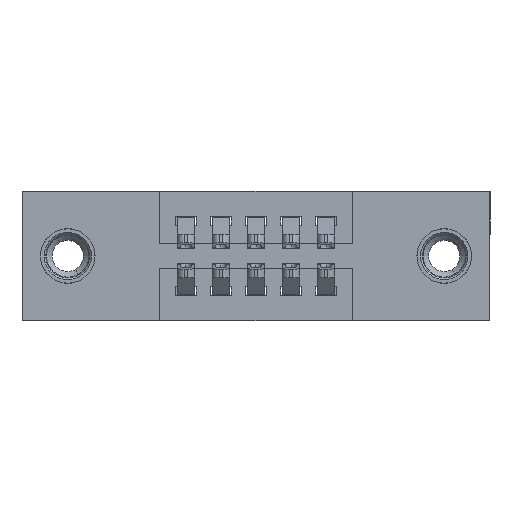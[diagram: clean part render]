
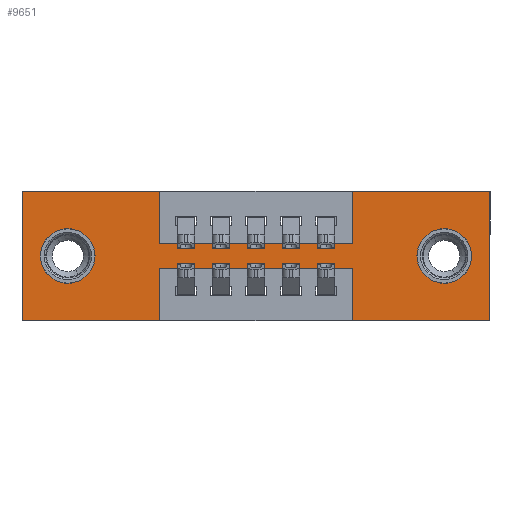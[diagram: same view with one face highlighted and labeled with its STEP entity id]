
A CAD part, front view. The second image highlights one B-rep face of the part: STEP entity #9651.
In plain terms, the highlighted planar face has unit normal (0, -1, 0).
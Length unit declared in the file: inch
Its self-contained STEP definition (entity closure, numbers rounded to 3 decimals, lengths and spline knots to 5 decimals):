
#229 = EDGE_LOOP ( 'NONE', ( #11366, #8792 ) ) ;
#254 = VERTEX_POINT ( 'NONE', #991 ) ;
#632 = FACE_OUTER_BOUND ( 'NONE', #6488, .T. ) ;
#671 = VECTOR ( 'NONE', #4247, 39.37008 ) ;
#933 = DIRECTION ( 'NONE',  ( -1., 0., 0. ) ) ;
#991 = CARTESIAN_POINT ( 'NONE',  ( 0.13, 0., -0.107 ) ) ;
#1004 = CARTESIAN_POINT ( 'NONE',  ( 0.3925, 0., -0.15 ) ) ;
#1120 = DIRECTION ( 'NONE',  ( 0., 1., 0. ) ) ;
#1125 = EDGE_CURVE ( 'NONE', #12646, #8550, #12252, .T. ) ;
#1458 = VERTEX_POINT ( 'NONE', #2628 ) ;
#1534 = ORIENTED_EDGE ( 'NONE', *, *, #6074, .F. ) ;
#1976 = VECTOR ( 'NONE', #12030, 39.37008 ) ;
#2078 = CARTESIAN_POINT ( 'NONE',  ( 0.13, 0., -0.185 ) ) ;
#2145 = LINE ( 'NONE', #2815, #13195 ) ;
#2158 = CARTESIAN_POINT ( 'NONE',  ( 0., 0., -0.37 ) ) ;
#2210 = PLANE ( 'NONE',  #7024 ) ;
#2267 = CARTESIAN_POINT ( 'NONE',  ( 0.9425, 0., -0.37 ) ) ;
#2303 = CARTESIAN_POINT ( 'NONE',  ( 1.205, 0., -0.185 ) ) ;
#2344 = ORIENTED_EDGE ( 'NONE', *, *, #8159, .F. ) ;
#2494 = VERTEX_POINT ( 'NONE', #3335 ) ;
#2552 = CARTESIAN_POINT ( 'NONE',  ( 0.13, 0., -0.185 ) ) ;
#2619 = CARTESIAN_POINT ( 'NONE',  ( 0.9425, 0., -0.37 ) ) ;
#2628 = CARTESIAN_POINT ( 'NONE',  ( 0.9425, 0., 0. ) ) ;
#2689 = CARTESIAN_POINT ( 'NONE',  ( 0., 0., -0.37 ) ) ;
#2693 = VECTOR ( 'NONE', #6007, 39.37008 ) ;
#2753 = ORIENTED_EDGE ( 'NONE', *, *, #3993, .F. ) ;
#2815 = CARTESIAN_POINT ( 'NONE',  ( 0.9425, 0., 0. ) ) ;
#2883 = CARTESIAN_POINT ( 'NONE',  ( 1.335, 0., -0.37 ) ) ;
#2893 = CARTESIAN_POINT ( 'NONE',  ( 0.13, 0., -0.263 ) ) ;
#2977 = VERTEX_POINT ( 'NONE', #6370 ) ;
#3029 = LINE ( 'NONE', #7100, #2693 ) ;
#3079 = VERTEX_POINT ( 'NONE', #12874 ) ;
#3143 = DIRECTION ( 'NONE',  ( 0., 0., 1. ) ) ;
#3152 = CARTESIAN_POINT ( 'NONE',  ( 0., 0., 0. ) ) ;
#3208 = CARTESIAN_POINT ( 'NONE',  ( 0.3925, 0., 0. ) ) ;
#3283 = LINE ( 'NONE', #7606, #5540 ) ;
#3298 = LINE ( 'NONE', #7542, #11921 ) ;
#3320 = DIRECTION ( 'NONE',  ( 0., 0., -1. ) ) ;
#3335 = CARTESIAN_POINT ( 'NONE',  ( 0.9425, 0., -0.22 ) ) ;
#3363 = DIRECTION ( 'NONE',  ( 0., 0., -1. ) ) ;
#3390 = VECTOR ( 'NONE', #10208, 39.37008 ) ;
#3630 = DIRECTION ( 'NONE',  ( 0., 0., 1. ) ) ;
#3690 = VERTEX_POINT ( 'NONE', #5334 ) ;
#3976 = VECTOR ( 'NONE', #13408, 39.37008 ) ;
#3981 = ORIENTED_EDGE ( 'NONE', *, *, #12559, .F. ) ;
#3993 = EDGE_CURVE ( 'NONE', #10356, #2977, #3029, .T. ) ;
#4084 = VERTEX_POINT ( 'NONE', #2883 ) ;
#4247 = DIRECTION ( 'NONE',  ( 0., 0., 1. ) ) ;
#4345 = VECTOR ( 'NONE', #7446, 39.37008 ) ;
#4351 = VECTOR ( 'NONE', #8367, 39.37008 ) ;
#4363 = VERTEX_POINT ( 'NONE', #2267 ) ;
#4379 = CARTESIAN_POINT ( 'NONE',  ( 0., 0., -0.37 ) ) ;
#4696 = LINE ( 'NONE', #10575, #4345 ) ;
#4722 = ORIENTED_EDGE ( 'NONE', *, *, #6990, .F. ) ;
#4725 = CARTESIAN_POINT ( 'NONE',  ( 1.205, 0., -0.263 ) ) ;
#5052 = DIRECTION ( 'NONE',  ( 0., 0., 1. ) ) ;
#5334 = CARTESIAN_POINT ( 'NONE',  ( 1.205, 0., -0.107 ) ) ;
#5540 = VECTOR ( 'NONE', #8664, 39.37008 ) ;
#5750 = VERTEX_POINT ( 'NONE', #2893 ) ;
#5808 = EDGE_CURVE ( 'NONE', #1458, #3079, #4696, .T. ) ;
#6007 = DIRECTION ( 'NONE',  ( 0., 0., -1. ) ) ;
#6074 = EDGE_CURVE ( 'NONE', #3079, #4084, #10572, .T. ) ;
#6370 = CARTESIAN_POINT ( 'NONE',  ( 0.3925, 0., -0.37 ) ) ;
#6488 = EDGE_LOOP ( 'NONE', ( #2753, #6684, #8919, #10282, #1534, #11613, #9801, #3981, #4722, #10330, #2344, #8836 ) ) ;
#6562 = LINE ( 'NONE', #3152, #671 ) ;
#6684 = ORIENTED_EDGE ( 'NONE', *, *, #11426, .F. ) ;
#6859 = FACE_BOUND ( 'NONE', #7692, .T. ) ;
#6865 = VERTEX_POINT ( 'NONE', #12658 ) ;
#6906 = LINE ( 'NONE', #2689, #3976 ) ;
#6990 = EDGE_CURVE ( 'NONE', #8550, #6865, #3283, .T. ) ;
#7009 = EDGE_CURVE ( 'NONE', #2977, #7177, #11235, .T. ) ;
#7024 = AXIS2_PLACEMENT_3D ( 'NONE', #4379, #9781, #3320 ) ;
#7100 = CARTESIAN_POINT ( 'NONE',  ( 0.3925, 0., -0.37 ) ) ;
#7177 = VERTEX_POINT ( 'NONE', #10061 ) ;
#7424 = CIRCLE ( 'NONE', #13664, 0.078 ) ;
#7446 = DIRECTION ( 'NONE',  ( 1., 0., 0. ) ) ;
#7542 = CARTESIAN_POINT ( 'NONE',  ( 0.3925, 0., -0.22 ) ) ;
#7606 = CARTESIAN_POINT ( 'NONE',  ( 0.3925, 0., 0. ) ) ;
#7692 = EDGE_LOOP ( 'NONE', ( #9797, #9050 ) ) ;
#7714 = CARTESIAN_POINT ( 'NONE',  ( 1.205, 0., -0.185 ) ) ;
#7761 = AXIS2_PLACEMENT_3D ( 'NONE', #2303, #9832, #3363 ) ;
#7773 = CARTESIAN_POINT ( 'NONE',  ( 0.3925, 0., -0.22 ) ) ;
#8093 = VERTEX_POINT ( 'NONE', #12670 ) ;
#8159 = EDGE_CURVE ( 'NONE', #7177, #12646, #6562, .T. ) ;
#8367 = DIRECTION ( 'NONE',  ( 1., 0., 0. ) ) ;
#8550 = VERTEX_POINT ( 'NONE', #3208 ) ;
#8664 = DIRECTION ( 'NONE',  ( 0., 0., -1. ) ) ;
#8775 = DIRECTION ( 'NONE',  ( 0., 0., -1. ) ) ;
#8792 = ORIENTED_EDGE ( 'NONE', *, *, #11991, .T. ) ;
#8836 = ORIENTED_EDGE ( 'NONE', *, *, #7009, .F. ) ;
#8919 = ORIENTED_EDGE ( 'NONE', *, *, #9882, .F. ) ;
#9050 = ORIENTED_EDGE ( 'NONE', *, *, #9533, .T. ) ;
#9165 = LINE ( 'NONE', #2619, #3390 ) ;
#9526 = LINE ( 'NONE', #1004, #12363 ) ;
#9527 = AXIS2_PLACEMENT_3D ( 'NONE', #2552, #10097, #3630 ) ;
#9533 = EDGE_CURVE ( 'NONE', #5750, #254, #13781, .T. ) ;
#9597 = DIRECTION ( 'NONE',  ( 0., 1., 0. ) ) ;
#9651 = ADVANCED_FACE ( 'NONE', ( #12170, #6859, #632 ), #2210, .T. ) ;
#9674 = EDGE_CURVE ( 'NONE', #3690, #13548, #11853, .T. ) ;
#9694 = DIRECTION ( 'NONE',  ( -1., 0., 0. ) ) ;
#9781 = DIRECTION ( 'NONE',  ( 0., -1., 0. ) ) ;
#9797 = ORIENTED_EDGE ( 'NONE', *, *, #13395, .T. ) ;
#9801 = ORIENTED_EDGE ( 'NONE', *, *, #11257, .F. ) ;
#9832 = DIRECTION ( 'NONE',  ( 0., 1., 0. ) ) ;
#9835 = CARTESIAN_POINT ( 'NONE',  ( 0., 0., 0. ) ) ;
#9882 = EDGE_CURVE ( 'NONE', #4363, #2494, #9165, .T. ) ;
#10061 = CARTESIAN_POINT ( 'NONE',  ( 0., 0., -0.37 ) ) ;
#10097 = DIRECTION ( 'NONE',  ( 0., 1., 0. ) ) ;
#10208 = DIRECTION ( 'NONE',  ( 0., 0., 1. ) ) ;
#10282 = ORIENTED_EDGE ( 'NONE', *, *, #11811, .F. ) ;
#10330 = ORIENTED_EDGE ( 'NONE', *, *, #1125, .F. ) ;
#10356 = VERTEX_POINT ( 'NONE', #7773 ) ;
#10572 = LINE ( 'NONE', #12991, #1976 ) ;
#10575 = CARTESIAN_POINT ( 'NONE',  ( 0., 0., 0. ) ) ;
#10853 = AXIS2_PLACEMENT_3D ( 'NONE', #2078, #9597, #3143 ) ;
#11235 = LINE ( 'NONE', #2158, #13656 ) ;
#11257 = EDGE_CURVE ( 'NONE', #8093, #1458, #2145, .T. ) ;
#11366 = ORIENTED_EDGE ( 'NONE', *, *, #9674, .T. ) ;
#11426 = EDGE_CURVE ( 'NONE', #2494, #10356, #3298, .T. ) ;
#11613 = ORIENTED_EDGE ( 'NONE', *, *, #5808, .F. ) ;
#11811 = EDGE_CURVE ( 'NONE', #4084, #4363, #6906, .T. ) ;
#11853 = CIRCLE ( 'NONE', #7761, 0.078 ) ;
#11921 = VECTOR ( 'NONE', #933, 39.37008 ) ;
#11991 = EDGE_CURVE ( 'NONE', #13548, #3690, #7424, .T. ) ;
#12030 = DIRECTION ( 'NONE',  ( 0., 0., -1. ) ) ;
#12170 = FACE_BOUND ( 'NONE', #229, .T. ) ;
#12252 = LINE ( 'NONE', #12797, #4351 ) ;
#12363 = VECTOR ( 'NONE', #12844, 39.37008 ) ;
#12559 = EDGE_CURVE ( 'NONE', #6865, #8093, #9526, .T. ) ;
#12646 = VERTEX_POINT ( 'NONE', #9835 ) ;
#12658 = CARTESIAN_POINT ( 'NONE',  ( 0.3925, 0., -0.15 ) ) ;
#12670 = CARTESIAN_POINT ( 'NONE',  ( 0.9425, 0., -0.15 ) ) ;
#12797 = CARTESIAN_POINT ( 'NONE',  ( 0., 0., 0. ) ) ;
#12844 = DIRECTION ( 'NONE',  ( 1., 0., 0. ) ) ;
#12874 = CARTESIAN_POINT ( 'NONE',  ( 1.335, 0., 0. ) ) ;
#12991 = CARTESIAN_POINT ( 'NONE',  ( 1.335, 0., 0. ) ) ;
#13195 = VECTOR ( 'NONE', #5052, 39.37008 ) ;
#13395 = EDGE_CURVE ( 'NONE', #254, #5750, #13948, .T. ) ;
#13408 = DIRECTION ( 'NONE',  ( -1., 0., 0. ) ) ;
#13548 = VERTEX_POINT ( 'NONE', #4725 ) ;
#13656 = VECTOR ( 'NONE', #9694, 39.37008 ) ;
#13664 = AXIS2_PLACEMENT_3D ( 'NONE', #7714, #1120, #8775 ) ;
#13781 = CIRCLE ( 'NONE', #10853, 0.078 ) ;
#13948 = CIRCLE ( 'NONE', #9527, 0.078 ) ;
